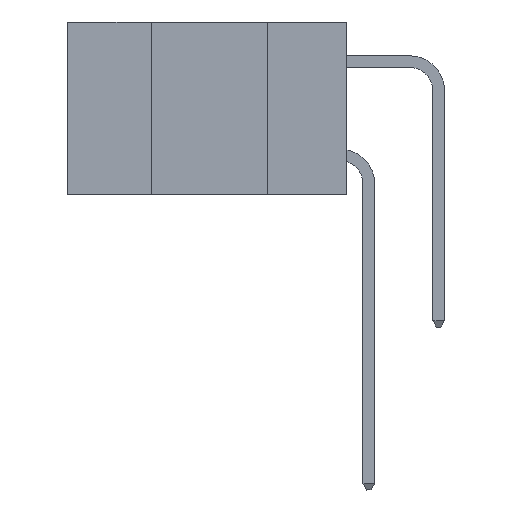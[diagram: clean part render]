
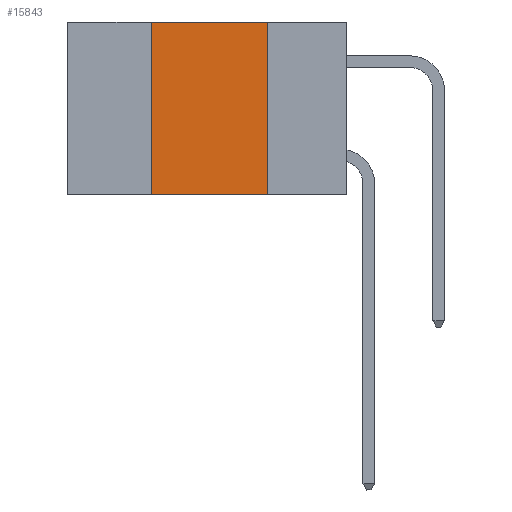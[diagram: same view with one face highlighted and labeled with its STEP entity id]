
A CAD part, left-side view. The second image highlights one B-rep face of the part: STEP entity #15843.
In plain terms, the highlighted planar face has unit normal (-1, 0, 0).
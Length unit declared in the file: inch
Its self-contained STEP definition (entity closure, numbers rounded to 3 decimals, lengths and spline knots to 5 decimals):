
#625 = VERTEX_POINT ( 'NONE', #13469 ) ;
#670 = VERTEX_POINT ( 'NONE', #3352 ) ;
#703 = LINE ( 'NONE', #5962, #18549 ) ;
#1358 = EDGE_LOOP ( 'NONE', ( #2253, #18455, #4152, #6285 ) ) ;
#1575 = LINE ( 'NONE', #6036, #6159 ) ;
#2253 = ORIENTED_EDGE ( 'NONE', *, *, #3394, .F. ) ;
#3352 = CARTESIAN_POINT ( 'NONE',  ( 0., 0.17, 0. ) ) ;
#3394 = EDGE_CURVE ( 'NONE', #670, #5692, #7071, .T. ) ;
#4152 = ORIENTED_EDGE ( 'NONE', *, *, #15849, .F. ) ;
#4245 = PLANE ( 'NONE',  #11163 ) ;
#5692 = VERTEX_POINT ( 'NONE', #9865 ) ;
#5962 = CARTESIAN_POINT ( 'NONE',  ( 0., 0.6, -0.37 ) ) ;
#6036 = CARTESIAN_POINT ( 'NONE',  ( 0., 0.42, 0. ) ) ;
#6159 = VECTOR ( 'NONE', #18135, 39.37008 ) ;
#6285 = ORIENTED_EDGE ( 'NONE', *, *, #19831, .T. ) ;
#7071 = LINE ( 'NONE', #17841, #10098 ) ;
#7695 = DIRECTION ( 'NONE',  ( 0., 0., -1. ) ) ;
#8066 = DIRECTION ( 'NONE',  ( 0., 0., -1. ) ) ;
#9469 = DIRECTION ( 'NONE',  ( 0., -1., 0. ) ) ;
#9865 = CARTESIAN_POINT ( 'NONE',  ( 0., 0.17, -0.37 ) ) ;
#9875 = CARTESIAN_POINT ( 'NONE',  ( 0., 0.42, 0. ) ) ;
#10098 = VECTOR ( 'NONE', #8066, 39.37008 ) ;
#10920 = CARTESIAN_POINT ( 'NONE',  ( 0., 0.6, 0. ) ) ;
#11163 = AXIS2_PLACEMENT_3D ( 'NONE', #16355, #18066, #7695 ) ;
#12646 = DIRECTION ( 'NONE',  ( 0., -1., 0. ) ) ;
#13469 = CARTESIAN_POINT ( 'NONE',  ( 0., 0.42, -0.37 ) ) ;
#13890 = EDGE_CURVE ( 'NONE', #19453, #670, #22190, .T. ) ;
#15408 = FACE_OUTER_BOUND ( 'NONE', #1358, .T. ) ;
#15843 = ADVANCED_FACE ( 'NONE', ( #15408 ), #4245, .F. ) ;
#15849 = EDGE_CURVE ( 'NONE', #625, #19453, #1575, .T. ) ;
#16355 = CARTESIAN_POINT ( 'NONE',  ( 0., 0.6, 0. ) ) ;
#17640 = VECTOR ( 'NONE', #12646, 39.37008 ) ;
#17841 = CARTESIAN_POINT ( 'NONE',  ( 0., 0.17, 0. ) ) ;
#18066 = DIRECTION ( 'NONE',  ( 1., 0., 0. ) ) ;
#18135 = DIRECTION ( 'NONE',  ( 0., 0., 1. ) ) ;
#18455 = ORIENTED_EDGE ( 'NONE', *, *, #13890, .F. ) ;
#18549 = VECTOR ( 'NONE', #9469, 39.37008 ) ;
#19453 = VERTEX_POINT ( 'NONE', #9875 ) ;
#19831 = EDGE_CURVE ( 'NONE', #625, #5692, #703, .T. ) ;
#22190 = LINE ( 'NONE', #10920, #17640 ) ;
